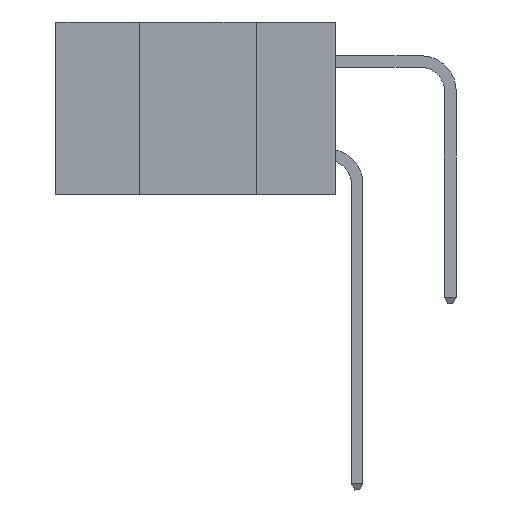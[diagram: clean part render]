
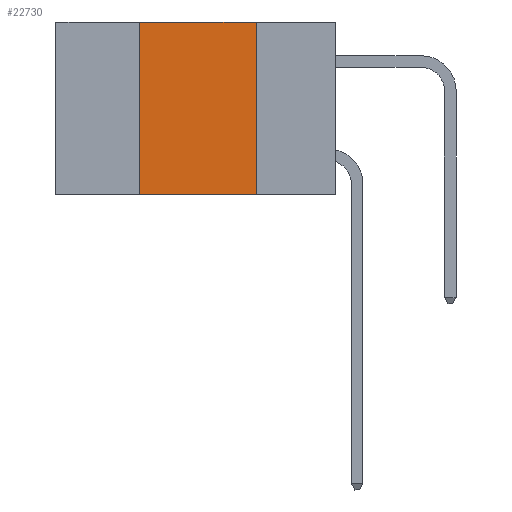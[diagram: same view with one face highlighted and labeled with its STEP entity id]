
A CAD part, left-side view. The second image highlights one B-rep face of the part: STEP entity #22730.
In plain terms, the highlighted planar face has unit normal (-1, 0, 0).
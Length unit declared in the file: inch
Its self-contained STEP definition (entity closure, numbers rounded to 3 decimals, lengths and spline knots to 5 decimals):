
#1755 = CARTESIAN_POINT ( 'NONE',  ( 0., 0.6, 0. ) ) ;
#2465 = EDGE_CURVE ( 'NONE', #25540, #38735, #28893, .T. ) ;
#2735 = VERTEX_POINT ( 'NONE', #34423 ) ;
#3818 = ORIENTED_EDGE ( 'NONE', *, *, #39225, .F. ) ;
#5465 = EDGE_CURVE ( 'NONE', #2735, #17108, #17422, .T. ) ;
#5569 = ORIENTED_EDGE ( 'NONE', *, *, #16881, .F. ) ;
#7077 = CARTESIAN_POINT ( 'NONE',  ( 0., 0.42, -0.37 ) ) ;
#11089 = VECTOR ( 'NONE', #17929, 39.37008 ) ;
#11889 = DIRECTION ( 'NONE',  ( 0., 0., 1. ) ) ;
#12303 = CARTESIAN_POINT ( 'NONE',  ( 0., 0.42, 0. ) ) ;
#15172 = VECTOR ( 'NONE', #16658, 39.37008 ) ;
#16658 = DIRECTION ( 'NONE',  ( 0., 0., -1. ) ) ;
#16881 = EDGE_CURVE ( 'NONE', #17108, #38735, #26409, .T. ) ;
#17108 = VERTEX_POINT ( 'NONE', #30595 ) ;
#17422 = LINE ( 'NONE', #39439, #11089 ) ;
#17929 = DIRECTION ( 'NONE',  ( 0., -1., 0. ) ) ;
#18095 = DIRECTION ( 'NONE',  ( 0., -1., 0. ) ) ;
#18507 = CARTESIAN_POINT ( 'NONE',  ( 0., 0.6, -0.37 ) ) ;
#20581 = DIRECTION ( 'NONE',  ( 0., 0., -1. ) ) ;
#20721 = DIRECTION ( 'NONE',  ( 1., 0., 0. ) ) ;
#20973 = FACE_OUTER_BOUND ( 'NONE', #25453, .T. ) ;
#22730 = ADVANCED_FACE ( 'NONE', ( #20973 ), #26719, .F. ) ;
#25453 = EDGE_LOOP ( 'NONE', ( #5569, #39943, #3818, #35608 ) ) ;
#25540 = VERTEX_POINT ( 'NONE', #7077 ) ;
#26409 = LINE ( 'NONE', #35399, #15172 ) ;
#26719 = PLANE ( 'NONE',  #29296 ) ;
#28893 = LINE ( 'NONE', #18507, #34260 ) ;
#29296 = AXIS2_PLACEMENT_3D ( 'NONE', #1755, #20721, #20581 ) ;
#30595 = CARTESIAN_POINT ( 'NONE',  ( 0., 0.17, 0. ) ) ;
#34021 = LINE ( 'NONE', #12303, #34516 ) ;
#34260 = VECTOR ( 'NONE', #18095, 39.37008 ) ;
#34423 = CARTESIAN_POINT ( 'NONE',  ( 0., 0.42, 0. ) ) ;
#34516 = VECTOR ( 'NONE', #11889, 39.37008 ) ;
#35399 = CARTESIAN_POINT ( 'NONE',  ( 0., 0.17, 0. ) ) ;
#35608 = ORIENTED_EDGE ( 'NONE', *, *, #2465, .T. ) ;
#37631 = CARTESIAN_POINT ( 'NONE',  ( 0., 0.17, -0.37 ) ) ;
#38735 = VERTEX_POINT ( 'NONE', #37631 ) ;
#39225 = EDGE_CURVE ( 'NONE', #25540, #2735, #34021, .T. ) ;
#39439 = CARTESIAN_POINT ( 'NONE',  ( 0., 0.6, 0. ) ) ;
#39943 = ORIENTED_EDGE ( 'NONE', *, *, #5465, .F. ) ;
